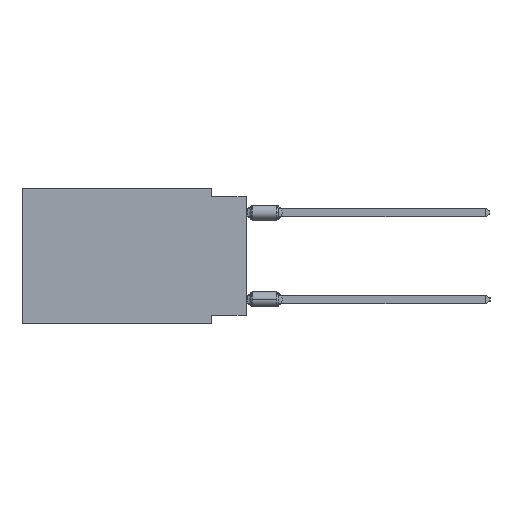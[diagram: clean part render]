
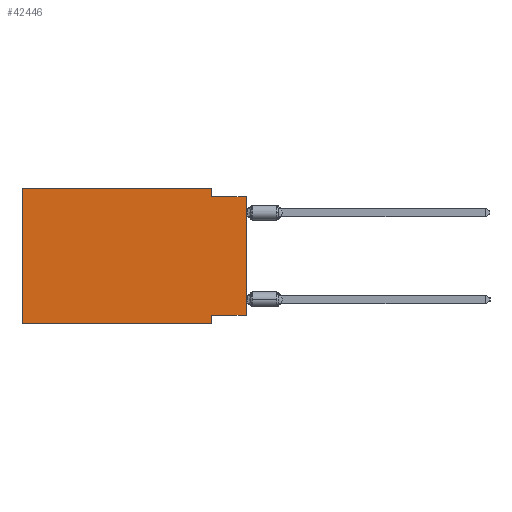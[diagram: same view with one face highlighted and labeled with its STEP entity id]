
A CAD part, left-side view. The second image highlights one B-rep face of the part: STEP entity #42446.
In plain terms, the highlighted planar face has unit normal (-1, 0, 0).
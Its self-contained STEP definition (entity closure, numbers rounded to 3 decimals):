
#472 = CARTESIAN_POINT ( 'NONE',  ( 0., 2.54, -9.271 ) ) ;
#778 = EDGE_CURVE ( 'NONE', #27477, #19191, #17539, .T. ) ;
#871 = EDGE_CURVE ( 'NONE', #41782, #20844, #5019, .T. ) ;
#883 = DIRECTION ( 'NONE',  ( 0., -1., 0. ) ) ;
#1408 = CARTESIAN_POINT ( 'NONE',  ( 0., 0., -0.635 ) ) ;
#2289 = VECTOR ( 'NONE', #31929, 1000. ) ;
#2570 = CARTESIAN_POINT ( 'NONE',  ( 0., 16.383, 0. ) ) ;
#3763 = EDGE_CURVE ( 'NONE', #21265, #19191, #43901, .T. ) ;
#4480 = LINE ( 'NONE', #43616, #15780 ) ;
#4664 = EDGE_CURVE ( 'NONE', #6247, #5626, #36694, .T. ) ;
#4955 = LINE ( 'NONE', #23091, #35716 ) ;
#5019 = LINE ( 'NONE', #43450, #21885 ) ;
#5045 = ORIENTED_EDGE ( 'NONE', *, *, #778, .F. ) ;
#5626 = VERTEX_POINT ( 'NONE', #45226 ) ;
#5637 = LINE ( 'NONE', #42143, #33603 ) ;
#5644 = CARTESIAN_POINT ( 'NONE',  ( 0., 16.383, 0. ) ) ;
#6088 = DIRECTION ( 'NONE',  ( 0., 0., 1. ) ) ;
#6247 = VERTEX_POINT ( 'NONE', #7919 ) ;
#6404 = CARTESIAN_POINT ( 'NONE',  ( 0., 2.54, -9.906 ) ) ;
#7919 = CARTESIAN_POINT ( 'NONE',  ( 0., 16.383, 0. ) ) ;
#8167 = EDGE_CURVE ( 'NONE', #5626, #41782, #4955, .T. ) ;
#12280 = EDGE_CURVE ( 'NONE', #46262, #20844, #5637, .T. ) ;
#12481 = DIRECTION ( 'NONE',  ( 0., 0., 1. ) ) ;
#13812 = ORIENTED_EDGE ( 'NONE', *, *, #3763, .T. ) ;
#15180 = EDGE_LOOP ( 'NONE', ( #30643, #27503, #35581, #15586, #23012, #13812, #5045, #28116 ) ) ;
#15586 = ORIENTED_EDGE ( 'NONE', *, *, #4664, .F. ) ;
#15780 = VECTOR ( 'NONE', #21933, 1000. ) ;
#17539 = LINE ( 'NONE', #28160, #2289 ) ;
#18031 = VECTOR ( 'NONE', #883, 1000. ) ;
#19191 = VERTEX_POINT ( 'NONE', #6404 ) ;
#19549 = DIRECTION ( 'NONE',  ( 1., 0., 0. ) ) ;
#19607 = EDGE_CURVE ( 'NONE', #21265, #6247, #33927, .T. ) ;
#20021 = DIRECTION ( 'NONE',  ( 0., 0., -1. ) ) ;
#20844 = VERTEX_POINT ( 'NONE', #1408 ) ;
#21265 = VERTEX_POINT ( 'NONE', #29426 ) ;
#21885 = VECTOR ( 'NONE', #25771, 1000. ) ;
#21933 = DIRECTION ( 'NONE',  ( 0., 1., 0. ) ) ;
#22917 = DIRECTION ( 'NONE',  ( 0., -1., 0. ) ) ;
#23012 = ORIENTED_EDGE ( 'NONE', *, *, #19607, .F. ) ;
#23091 = CARTESIAN_POINT ( 'NONE',  ( 0., 2.54, 0. ) ) ;
#23546 = PLANE ( 'NONE',  #32490 ) ;
#23777 = FACE_OUTER_BOUND ( 'NONE', #15180, .T. ) ;
#25771 = DIRECTION ( 'NONE',  ( 0., -1., 0. ) ) ;
#26075 = CARTESIAN_POINT ( 'NONE',  ( 0., 0., -9.271 ) ) ;
#27326 = DIRECTION ( 'NONE',  ( 0., 0., -1. ) ) ;
#27477 = VERTEX_POINT ( 'NONE', #472 ) ;
#27503 = ORIENTED_EDGE ( 'NONE', *, *, #871, .F. ) ;
#28116 = ORIENTED_EDGE ( 'NONE', *, *, #40359, .F. ) ;
#28160 = CARTESIAN_POINT ( 'NONE',  ( 0., 2.54, -9.906 ) ) ;
#29187 = CARTESIAN_POINT ( 'NONE',  ( 0., 16.383, 0. ) ) ;
#29426 = CARTESIAN_POINT ( 'NONE',  ( 0., 16.383, -9.906 ) ) ;
#30643 = ORIENTED_EDGE ( 'NONE', *, *, #12280, .T. ) ;
#31929 = DIRECTION ( 'NONE',  ( 0., 0., -1. ) ) ;
#32490 = AXIS2_PLACEMENT_3D ( 'NONE', #5644, #19549, #20021 ) ;
#32846 = CARTESIAN_POINT ( 'NONE',  ( 0., 16.383, -9.906 ) ) ;
#33603 = VECTOR ( 'NONE', #6088, 1000. ) ;
#33927 = LINE ( 'NONE', #2570, #34026 ) ;
#34026 = VECTOR ( 'NONE', #12481, 1000. ) ;
#35581 = ORIENTED_EDGE ( 'NONE', *, *, #8167, .F. ) ;
#35716 = VECTOR ( 'NONE', #27326, 1000. ) ;
#36694 = LINE ( 'NONE', #29187, #18031 ) ;
#37549 = VECTOR ( 'NONE', #22917, 1000. ) ;
#39441 = CARTESIAN_POINT ( 'NONE',  ( 0., 2.54, -0.635 ) ) ;
#40359 = EDGE_CURVE ( 'NONE', #46262, #27477, #4480, .T. ) ;
#41782 = VERTEX_POINT ( 'NONE', #39441 ) ;
#42143 = CARTESIAN_POINT ( 'NONE',  ( 0., 0., 0. ) ) ;
#42446 = ADVANCED_FACE ( 'NONE', ( #23777 ), #23546, .F. ) ;
#43450 = CARTESIAN_POINT ( 'NONE',  ( 0., 0., -0.635 ) ) ;
#43616 = CARTESIAN_POINT ( 'NONE',  ( 0., 0., -9.271 ) ) ;
#43901 = LINE ( 'NONE', #32846, #37549 ) ;
#45226 = CARTESIAN_POINT ( 'NONE',  ( 0., 2.54, 0. ) ) ;
#46262 = VERTEX_POINT ( 'NONE', #26075 ) ;
